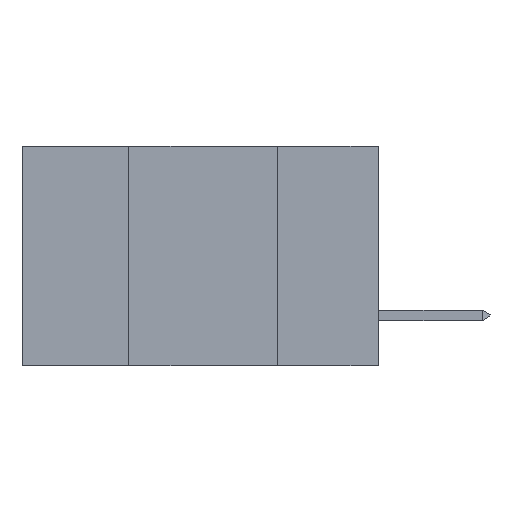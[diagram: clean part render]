
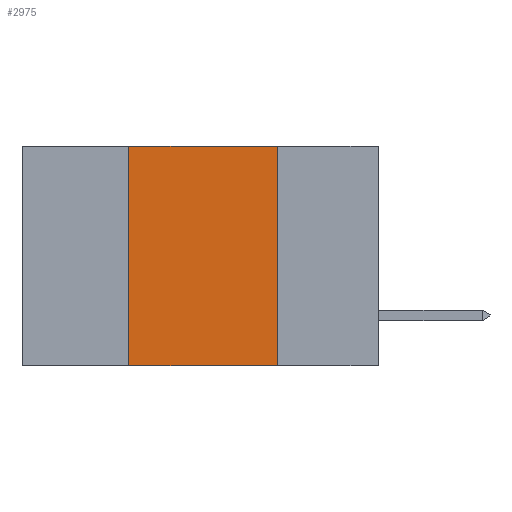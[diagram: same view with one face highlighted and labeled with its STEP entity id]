
A CAD part, left-side view. The second image highlights one B-rep face of the part: STEP entity #2975.
In plain terms, the highlighted planar face has unit normal (-1, 0, 0).
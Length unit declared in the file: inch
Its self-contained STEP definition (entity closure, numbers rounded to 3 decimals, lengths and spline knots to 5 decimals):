
#148 = CARTESIAN_POINT ( 'NONE',  ( 0., 0.17, -0.37 ) ) ;
#1134 = VECTOR ( 'NONE', #9533, 39.37008 ) ;
#1591 = VECTOR ( 'NONE', #2624, 39.37008 ) ;
#1684 = EDGE_CURVE ( 'NONE', #9490, #2270, #8862, .T. ) ;
#1849 = EDGE_CURVE ( 'NONE', #2270, #10876, #8046, .T. ) ;
#2082 = ORIENTED_EDGE ( 'NONE', *, *, #8432, .T. ) ;
#2177 = FACE_OUTER_BOUND ( 'NONE', #10348, .T. ) ;
#2270 = VERTEX_POINT ( 'NONE', #10201 ) ;
#2464 = CARTESIAN_POINT ( 'NONE',  ( 0., 0.6, -0.37 ) ) ;
#2624 = DIRECTION ( 'NONE',  ( 0., -1., 0. ) ) ;
#2975 = ADVANCED_FACE ( 'NONE', ( #2177 ), #10022, .F. ) ;
#2982 = CARTESIAN_POINT ( 'NONE',  ( 0., 0.42, 0. ) ) ;
#3652 = ORIENTED_EDGE ( 'NONE', *, *, #1849, .F. ) ;
#3828 = ORIENTED_EDGE ( 'NONE', *, *, #7931, .F. ) ;
#4704 = CARTESIAN_POINT ( 'NONE',  ( 0., 0.42, -0.37 ) ) ;
#4919 = CARTESIAN_POINT ( 'NONE',  ( 0., 0.6, 0. ) ) ;
#5101 = CARTESIAN_POINT ( 'NONE',  ( 0., 0.6, 0. ) ) ;
#5228 = CARTESIAN_POINT ( 'NONE',  ( 0., 0.17, 0. ) ) ;
#6042 = VERTEX_POINT ( 'NONE', #148 ) ;
#6315 = DIRECTION ( 'NONE',  ( 0., 0., 1. ) ) ;
#6320 = VECTOR ( 'NONE', #6315, 39.37008 ) ;
#6501 = AXIS2_PLACEMENT_3D ( 'NONE', #4919, #7496, #9256 ) ;
#6814 = DIRECTION ( 'NONE',  ( 0., -1., 0. ) ) ;
#7496 = DIRECTION ( 'NONE',  ( 1., 0., 0. ) ) ;
#7664 = ORIENTED_EDGE ( 'NONE', *, *, #1684, .F. ) ;
#7713 = LINE ( 'NONE', #5228, #1134 ) ;
#7931 = EDGE_CURVE ( 'NONE', #10876, #6042, #7713, .T. ) ;
#8046 = LINE ( 'NONE', #5101, #1591 ) ;
#8207 = CARTESIAN_POINT ( 'NONE',  ( 0., 0.17, 0. ) ) ;
#8234 = VECTOR ( 'NONE', #6814, 39.37008 ) ;
#8432 = EDGE_CURVE ( 'NONE', #9490, #6042, #9486, .T. ) ;
#8862 = LINE ( 'NONE', #2982, #6320 ) ;
#9256 = DIRECTION ( 'NONE',  ( 0., 0., -1. ) ) ;
#9486 = LINE ( 'NONE', #2464, #8234 ) ;
#9490 = VERTEX_POINT ( 'NONE', #4704 ) ;
#9533 = DIRECTION ( 'NONE',  ( 0., 0., -1. ) ) ;
#10022 = PLANE ( 'NONE',  #6501 ) ;
#10201 = CARTESIAN_POINT ( 'NONE',  ( 0., 0.42, 0. ) ) ;
#10348 = EDGE_LOOP ( 'NONE', ( #3828, #3652, #7664, #2082 ) ) ;
#10876 = VERTEX_POINT ( 'NONE', #8207 ) ;
